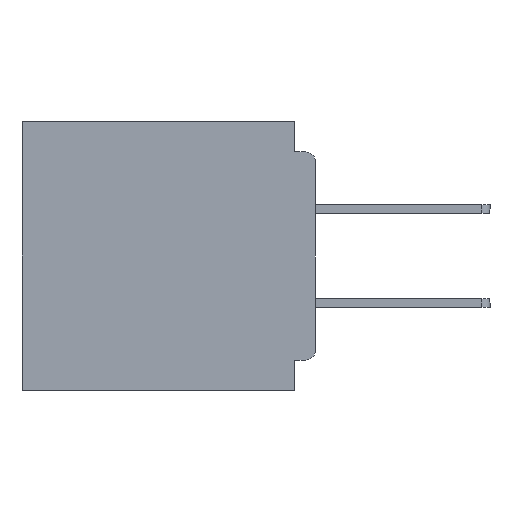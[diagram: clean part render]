
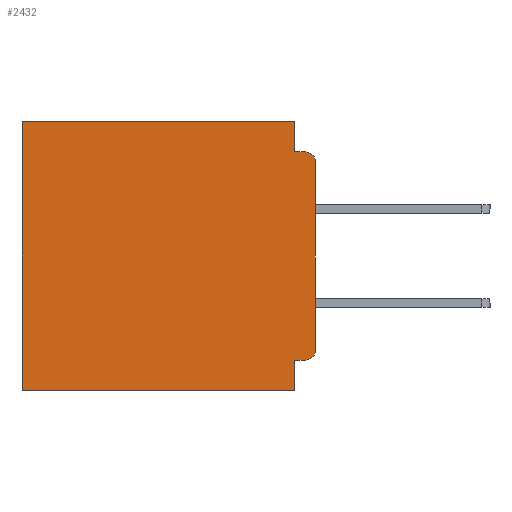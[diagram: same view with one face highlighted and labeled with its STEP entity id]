
A CAD part, left-side view. The second image highlights one B-rep face of the part: STEP entity #2432.
In plain terms, the highlighted planar face has unit normal (-1, 0, 0).
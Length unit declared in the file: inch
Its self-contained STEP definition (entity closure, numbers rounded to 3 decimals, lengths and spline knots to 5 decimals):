
#1434 = CARTESIAN_POINT ( 'NONE',  ( 0.3, 0.031, -0.4 ) ) ;
#1806 = LINE ( 'NONE', #3435, #34455 ) ;
#2432 = ADVANCED_FACE ( 'NONE', ( #35926 ), #23953, .F. ) ;
#3101 = CARTESIAN_POINT ( 'NONE',  ( 0.3, 0., -0.045 ) ) ;
#3435 = CARTESIAN_POINT ( 'NONE',  ( 0.3, 0.031, 0. ) ) ;
#4295 = LINE ( 'NONE', #59941, #52298 ) ;
#4415 = VERTEX_POINT ( 'NONE', #26946 ) ;
#4527 = VECTOR ( 'NONE', #35554, 39.37008 ) ;
#4533 = AXIS2_PLACEMENT_3D ( 'NONE', #17210, #49737, #21858 ) ;
#4578 = CIRCLE ( 'NONE', #14241, 0.015 ) ;
#4823 = EDGE_CURVE ( 'NONE', #50447, #5000, #6212, .T. ) ;
#5000 = VERTEX_POINT ( 'NONE', #32128 ) ;
#6088 = EDGE_CURVE ( 'NONE', #26021, #46582, #1806, .T. ) ;
#6112 = VERTEX_POINT ( 'NONE', #50145 ) ;
#6212 = LINE ( 'NONE', #53973, #29431 ) ;
#6884 = CARTESIAN_POINT ( 'NONE',  ( 0.3, 0.015, -0.045 ) ) ;
#7313 = EDGE_CURVE ( 'NONE', #46582, #27367, #15453, .T. ) ;
#7486 = LINE ( 'NONE', #1434, #29220 ) ;
#7584 = ORIENTED_EDGE ( 'NONE', *, *, #18167, .T. ) ;
#7824 = VERTEX_POINT ( 'NONE', #25339 ) ;
#8672 = AXIS2_PLACEMENT_3D ( 'NONE', #37156, #16039, #24069 ) ;
#8858 = EDGE_CURVE ( 'NONE', #4415, #6112, #31184, .T. ) ;
#9713 = ORIENTED_EDGE ( 'NONE', *, *, #4823, .F. ) ;
#9946 = EDGE_CURVE ( 'NONE', #26021, #30415, #4295, .T. ) ;
#10930 = CARTESIAN_POINT ( 'NONE',  ( 0.3, 0.031, 0. ) ) ;
#12116 = CARTESIAN_POINT ( 'NONE',  ( 0.3, 0.015, -0.34 ) ) ;
#13683 = EDGE_CURVE ( 'NONE', #6112, #19116, #7486, .T. ) ;
#14241 = AXIS2_PLACEMENT_3D ( 'NONE', #12116, #44579, #16745 ) ;
#15453 = LINE ( 'NONE', #3101, #4527 ) ;
#16039 = DIRECTION ( 'NONE',  ( 1., 0., 0. ) ) ;
#16745 = DIRECTION ( 'NONE',  ( 0., 0., -1. ) ) ;
#17210 = CARTESIAN_POINT ( 'NONE',  ( 0.3, 0.015, -0.06 ) ) ;
#17425 = DIRECTION ( 'NONE',  ( 0., 0., -1. ) ) ;
#18167 = EDGE_CURVE ( 'NONE', #4415, #5000, #4578, .T. ) ;
#19116 = VERTEX_POINT ( 'NONE', #42420 ) ;
#19138 = ORIENTED_EDGE ( 'NONE', *, *, #9946, .T. ) ;
#20031 = DIRECTION ( 'NONE',  ( 0., 0., -1. ) ) ;
#21858 = DIRECTION ( 'NONE',  ( 0., 0., -1. ) ) ;
#22919 = DIRECTION ( 'NONE',  ( 0., 1., 0. ) ) ;
#23953 = PLANE ( 'NONE',  #8672 ) ;
#24069 = DIRECTION ( 'NONE',  ( 0., 0., -1. ) ) ;
#25339 = CARTESIAN_POINT ( 'NONE',  ( 0.3, 0.437, -0.4 ) ) ;
#25496 = ORIENTED_EDGE ( 'NONE', *, *, #6088, .F. ) ;
#25509 = CARTESIAN_POINT ( 'NONE',  ( 0.3, 0., -0.4 ) ) ;
#25583 = EDGE_CURVE ( 'NONE', #19116, #7824, #40423, .T. ) ;
#26021 = VERTEX_POINT ( 'NONE', #10930 ) ;
#26946 = CARTESIAN_POINT ( 'NONE',  ( 0.3, 0.015, -0.355 ) ) ;
#27367 = VERTEX_POINT ( 'NONE', #6884 ) ;
#28384 = ORIENTED_EDGE ( 'NONE', *, *, #55697, .T. ) ;
#29106 = CARTESIAN_POINT ( 'NONE',  ( 0.3, 0., -0.355 ) ) ;
#29220 = VECTOR ( 'NONE', #43273, 39.37008 ) ;
#29431 = VECTOR ( 'NONE', #58940, 39.37008 ) ;
#30177 = DIRECTION ( 'NONE',  ( 0., 1., 0. ) ) ;
#30415 = VERTEX_POINT ( 'NONE', #46599 ) ;
#31184 = LINE ( 'NONE', #29106, #40634 ) ;
#32128 = CARTESIAN_POINT ( 'NONE',  ( 0.3, 0., -0.34 ) ) ;
#33820 = CARTESIAN_POINT ( 'NONE',  ( 0.3, 0.437, -0.4 ) ) ;
#34455 = VECTOR ( 'NONE', #17425, 39.37008 ) ;
#34476 = CARTESIAN_POINT ( 'NONE',  ( 0.3, 0.031, -0.045 ) ) ;
#35554 = DIRECTION ( 'NONE',  ( 0., -1., 0. ) ) ;
#35926 = FACE_OUTER_BOUND ( 'NONE', #47028, .T. ) ;
#37156 = CARTESIAN_POINT ( 'NONE',  ( 0.3, 0., -0.4 ) ) ;
#40423 = LINE ( 'NONE', #25509, #49912 ) ;
#40634 = VECTOR ( 'NONE', #47635, 39.37008 ) ;
#41834 = LINE ( 'NONE', #33820, #52788 ) ;
#42420 = CARTESIAN_POINT ( 'NONE',  ( 0.3, 0.031, -0.4 ) ) ;
#42801 = ORIENTED_EDGE ( 'NONE', *, *, #8858, .F. ) ;
#43273 = DIRECTION ( 'NONE',  ( 0., 0., -1. ) ) ;
#44579 = DIRECTION ( 'NONE',  ( -1., 0., 0. ) ) ;
#44757 = CARTESIAN_POINT ( 'NONE',  ( 0.3, 0., -0.06 ) ) ;
#46582 = VERTEX_POINT ( 'NONE', #34476 ) ;
#46599 = CARTESIAN_POINT ( 'NONE',  ( 0.3, 0.437, 0. ) ) ;
#47028 = EDGE_LOOP ( 'NONE', ( #9713, #47880, #58734, #25496, #19138, #28384, #48056, #48389, #42801, #7584 ) ) ;
#47635 = DIRECTION ( 'NONE',  ( 0., 1., 0. ) ) ;
#47880 = ORIENTED_EDGE ( 'NONE', *, *, #58005, .T. ) ;
#48056 = ORIENTED_EDGE ( 'NONE', *, *, #25583, .F. ) ;
#48389 = ORIENTED_EDGE ( 'NONE', *, *, #13683, .F. ) ;
#49737 = DIRECTION ( 'NONE',  ( -1., 0., 0. ) ) ;
#49912 = VECTOR ( 'NONE', #30177, 39.37008 ) ;
#50145 = CARTESIAN_POINT ( 'NONE',  ( 0.3, 0.031, -0.355 ) ) ;
#50447 = VERTEX_POINT ( 'NONE', #44757 ) ;
#51038 = CIRCLE ( 'NONE', #4533, 0.015 ) ;
#52298 = VECTOR ( 'NONE', #22919, 39.37008 ) ;
#52788 = VECTOR ( 'NONE', #20031, 39.37008 ) ;
#53973 = CARTESIAN_POINT ( 'NONE',  ( 0.3, 0., -0.4 ) ) ;
#55697 = EDGE_CURVE ( 'NONE', #30415, #7824, #41834, .T. ) ;
#58005 = EDGE_CURVE ( 'NONE', #50447, #27367, #51038, .T. ) ;
#58734 = ORIENTED_EDGE ( 'NONE', *, *, #7313, .F. ) ;
#58940 = DIRECTION ( 'NONE',  ( 0., 0., -1. ) ) ;
#59941 = CARTESIAN_POINT ( 'NONE',  ( 0.3, 0., 0. ) ) ;
